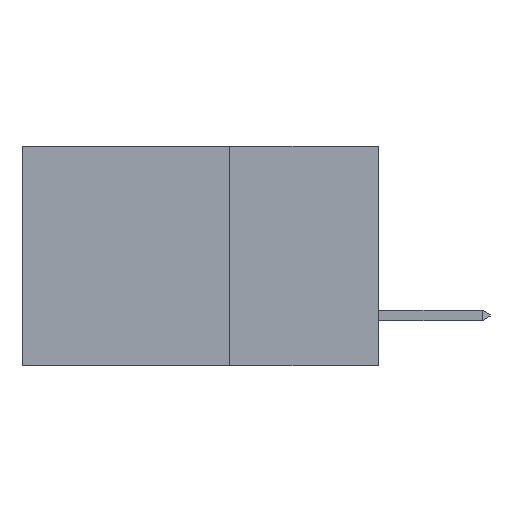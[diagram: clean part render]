
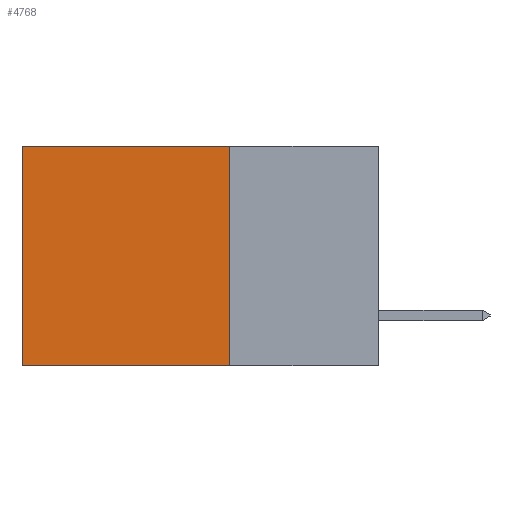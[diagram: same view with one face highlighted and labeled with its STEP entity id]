
A CAD part, left-side view. The second image highlights one B-rep face of the part: STEP entity #4768.
In plain terms, the highlighted planar face has unit normal (-1, 0, 0).
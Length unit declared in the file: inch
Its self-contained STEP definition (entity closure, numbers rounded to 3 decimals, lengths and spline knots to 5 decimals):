
#215 = DIRECTION ( 'NONE',  ( 0., 0., -1. ) ) ;
#1041 = CARTESIAN_POINT ( 'NONE',  ( 0.2615, 0.6, 0. ) ) ;
#1471 = VECTOR ( 'NONE', #215, 39.37008 ) ;
#1555 = EDGE_CURVE ( 'NONE', #8023, #6915, #8345, .T. ) ;
#1615 = DIRECTION ( 'NONE',  ( 0., 0., -1. ) ) ;
#1654 = DIRECTION ( 'NONE',  ( 1., 0., 0. ) ) ;
#1666 = CARTESIAN_POINT ( 'NONE',  ( 0.2615, 0.25, -0.37 ) ) ;
#1722 = EDGE_LOOP ( 'NONE', ( #7977, #4965, #4020, #8097 ) ) ;
#1735 = PLANE ( 'NONE',  #2418 ) ;
#2418 = AXIS2_PLACEMENT_3D ( 'NONE', #1666, #1654, #1615 ) ;
#2537 = LINE ( 'NONE', #3021, #3769 ) ;
#2548 = CARTESIAN_POINT ( 'NONE',  ( 0.2615, 0.25, 0. ) ) ;
#2886 = FACE_OUTER_BOUND ( 'NONE', #1722, .T. ) ;
#2986 = DIRECTION ( 'NONE',  ( 0., 0., -1. ) ) ;
#3021 = CARTESIAN_POINT ( 'NONE',  ( 0.2615, 0.6, -0.37 ) ) ;
#3769 = VECTOR ( 'NONE', #2986, 39.37008 ) ;
#3939 = VERTEX_POINT ( 'NONE', #8868 ) ;
#4020 = ORIENTED_EDGE ( 'NONE', *, *, #7485, .F. ) ;
#4462 = CARTESIAN_POINT ( 'NONE',  ( 0.2615, 0.25, -0.37 ) ) ;
#4768 = ADVANCED_FACE ( 'NONE', ( #2886 ), #1735, .F. ) ;
#4965 = ORIENTED_EDGE ( 'NONE', *, *, #6855, .F. ) ;
#5135 = DIRECTION ( 'NONE',  ( 0., 1., 0. ) ) ;
#5347 = VECTOR ( 'NONE', #5135, 39.37008 ) ;
#5647 = CARTESIAN_POINT ( 'NONE',  ( 0.2615, 0.6, -0.37 ) ) ;
#5708 = CARTESIAN_POINT ( 'NONE',  ( 0.2615, 0.25, 0. ) ) ;
#6063 = VERTEX_POINT ( 'NONE', #5647 ) ;
#6120 = DIRECTION ( 'NONE',  ( 0., 1., 0. ) ) ;
#6373 = EDGE_CURVE ( 'NONE', #6915, #6063, #2537, .T. ) ;
#6502 = VECTOR ( 'NONE', #6120, 39.37008 ) ;
#6855 = EDGE_CURVE ( 'NONE', #3939, #6063, #7389, .T. ) ;
#6915 = VERTEX_POINT ( 'NONE', #1041 ) ;
#7389 = LINE ( 'NONE', #4462, #5347 ) ;
#7485 = EDGE_CURVE ( 'NONE', #8023, #3939, #8801, .T. ) ;
#7977 = ORIENTED_EDGE ( 'NONE', *, *, #6373, .T. ) ;
#8023 = VERTEX_POINT ( 'NONE', #5708 ) ;
#8097 = ORIENTED_EDGE ( 'NONE', *, *, #1555, .T. ) ;
#8345 = LINE ( 'NONE', #2548, #6502 ) ;
#8485 = CARTESIAN_POINT ( 'NONE',  ( 0.2615, 0.25, -0.37 ) ) ;
#8801 = LINE ( 'NONE', #8485, #1471 ) ;
#8868 = CARTESIAN_POINT ( 'NONE',  ( 0.2615, 0.25, -0.37 ) ) ;
